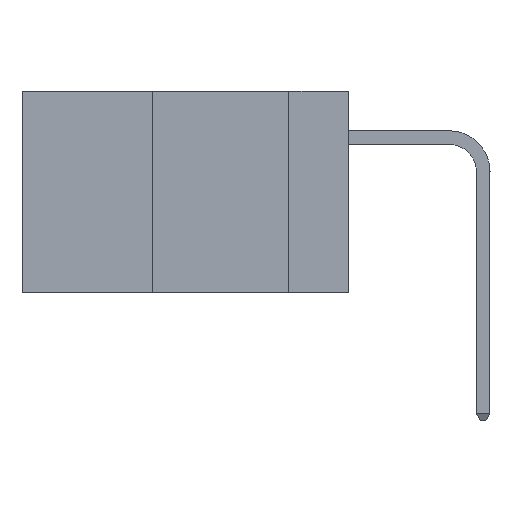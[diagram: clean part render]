
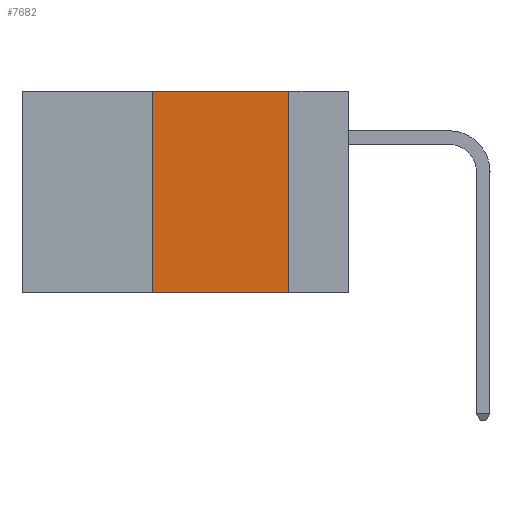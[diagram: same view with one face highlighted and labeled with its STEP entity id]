
A CAD part, left-side view. The second image highlights one B-rep face of the part: STEP entity #7682.
In plain terms, the highlighted planar face has unit normal (-1, 0, 0).
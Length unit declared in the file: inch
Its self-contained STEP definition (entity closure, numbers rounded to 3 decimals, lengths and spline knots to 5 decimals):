
#1164 = VERTEX_POINT ( 'NONE', #19710 ) ;
#2423 = ORIENTED_EDGE ( 'NONE', *, *, #12639, .F. ) ;
#3573 = DIRECTION ( 'NONE',  ( 1., 0., 0. ) ) ;
#5300 = ORIENTED_EDGE ( 'NONE', *, *, #15224, .T. ) ;
#6263 = VECTOR ( 'NONE', #12763, 39.37008 ) ;
#6984 = ORIENTED_EDGE ( 'NONE', *, *, #15173, .F. ) ;
#7682 = ADVANCED_FACE ( 'NONE', ( #9681 ), #23917, .F. ) ;
#7951 = CARTESIAN_POINT ( 'NONE',  ( 0., 0.6, -0.37 ) ) ;
#8318 = DIRECTION ( 'NONE',  ( 0., -1., 0. ) ) ;
#8847 = LINE ( 'NONE', #31950, #33317 ) ;
#9498 = DIRECTION ( 'NONE',  ( 0., 0., -1. ) ) ;
#9681 = FACE_OUTER_BOUND ( 'NONE', #18454, .T. ) ;
#9804 = VECTOR ( 'NONE', #8318, 39.37008 ) ;
#11460 = VERTEX_POINT ( 'NONE', #20300 ) ;
#12639 = EDGE_CURVE ( 'NONE', #11460, #30408, #8847, .T. ) ;
#12727 = CARTESIAN_POINT ( 'NONE',  ( 0., 0.11, -0.37 ) ) ;
#12763 = DIRECTION ( 'NONE',  ( 0., 0., 1. ) ) ;
#15131 = VECTOR ( 'NONE', #35017, 39.37008 ) ;
#15173 = EDGE_CURVE ( 'NONE', #1164, #11460, #29578, .T. ) ;
#15224 = EDGE_CURVE ( 'NONE', #1164, #33715, #30510, .T. ) ;
#17134 = EDGE_CURVE ( 'NONE', #30408, #33715, #34474, .T. ) ;
#18454 = EDGE_LOOP ( 'NONE', ( #36394, #2423, #6984, #5300 ) ) ;
#18523 = AXIS2_PLACEMENT_3D ( 'NONE', #26337, #3573, #9498 ) ;
#19710 = CARTESIAN_POINT ( 'NONE',  ( 0., 0.36, -0.37 ) ) ;
#20300 = CARTESIAN_POINT ( 'NONE',  ( 0., 0.36, 0. ) ) ;
#23917 = PLANE ( 'NONE',  #18523 ) ;
#26337 = CARTESIAN_POINT ( 'NONE',  ( 0., 0.6, 0. ) ) ;
#26817 = CARTESIAN_POINT ( 'NONE',  ( 0., 0.36, 0. ) ) ;
#29023 = CARTESIAN_POINT ( 'NONE',  ( 0., 0.11, 0. ) ) ;
#29578 = LINE ( 'NONE', #26817, #6263 ) ;
#30408 = VERTEX_POINT ( 'NONE', #29023 ) ;
#30510 = LINE ( 'NONE', #7951, #9804 ) ;
#31950 = CARTESIAN_POINT ( 'NONE',  ( 0., 0.6, 0. ) ) ;
#33317 = VECTOR ( 'NONE', #34179, 39.37008 ) ;
#33715 = VERTEX_POINT ( 'NONE', #12727 ) ;
#34179 = DIRECTION ( 'NONE',  ( 0., -1., 0. ) ) ;
#34474 = LINE ( 'NONE', #34841, #15131 ) ;
#34841 = CARTESIAN_POINT ( 'NONE',  ( 0., 0.11, 0. ) ) ;
#35017 = DIRECTION ( 'NONE',  ( 0., 0., -1. ) ) ;
#36394 = ORIENTED_EDGE ( 'NONE', *, *, #17134, .F. ) ;
